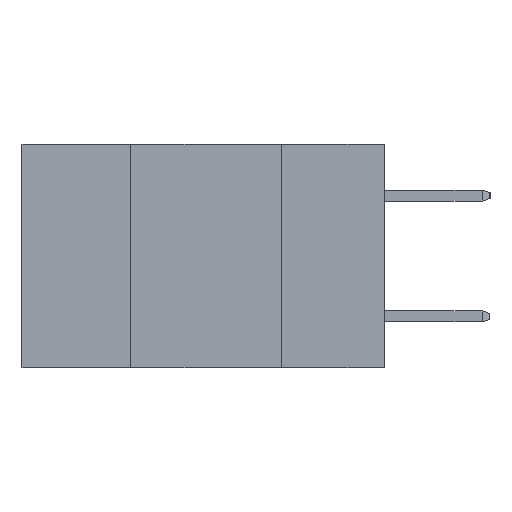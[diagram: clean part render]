
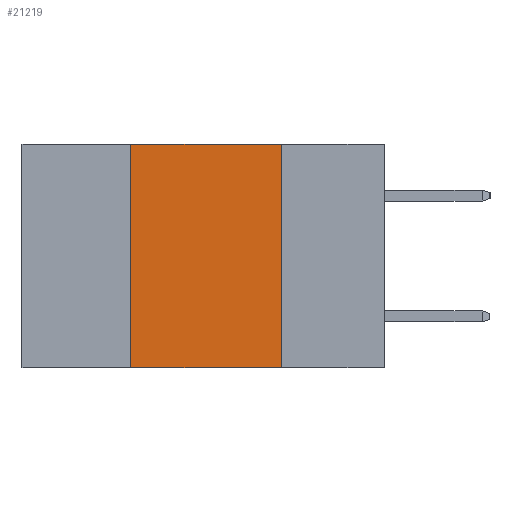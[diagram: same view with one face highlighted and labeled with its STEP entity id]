
A CAD part, left-side view. The second image highlights one B-rep face of the part: STEP entity #21219.
In plain terms, the highlighted planar face has unit normal (-1, 0, 0).
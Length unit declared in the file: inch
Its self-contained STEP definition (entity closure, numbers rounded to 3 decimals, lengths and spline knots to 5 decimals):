
#1709 = CARTESIAN_POINT ( 'NONE',  ( 0., 0.42, -0.37 ) ) ;
#1717 = VECTOR ( 'NONE', #9389, 39.37008 ) ;
#1955 = LINE ( 'NONE', #6246, #3697 ) ;
#2546 = CARTESIAN_POINT ( 'NONE',  ( 0., 0.42, -0.37 ) ) ;
#2912 = EDGE_CURVE ( 'NONE', #18429, #22947, #5205, .T. ) ;
#3544 = ORIENTED_EDGE ( 'NONE', *, *, #7092, .F. ) ;
#3697 = VECTOR ( 'NONE', #4230, 39.37008 ) ;
#3703 = CARTESIAN_POINT ( 'NONE',  ( 0., 0.17, -0.37 ) ) ;
#4230 = DIRECTION ( 'NONE',  ( 0., -1., 0. ) ) ;
#5205 = LINE ( 'NONE', #1709, #26503 ) ;
#5547 = AXIS2_PLACEMENT_3D ( 'NONE', #24723, #12268, #7936 ) ;
#6246 = CARTESIAN_POINT ( 'NONE',  ( 0., 0.6, -0.37 ) ) ;
#6876 = VERTEX_POINT ( 'NONE', #11028 ) ;
#7092 = EDGE_CURVE ( 'NONE', #6876, #13801, #21969, .T. ) ;
#7185 = EDGE_LOOP ( 'NONE', ( #3544, #21070, #16574, #25430 ) ) ;
#7936 = DIRECTION ( 'NONE',  ( 0., 0., -1. ) ) ;
#9389 = DIRECTION ( 'NONE',  ( 0., 0., -1. ) ) ;
#9823 = EDGE_CURVE ( 'NONE', #18429, #13801, #1955, .T. ) ;
#10939 = CARTESIAN_POINT ( 'NONE',  ( 0., 0.17, -0.37 ) ) ;
#11028 = CARTESIAN_POINT ( 'NONE',  ( 0., 0.17, 0. ) ) ;
#12135 = PLANE ( 'NONE',  #5547 ) ;
#12268 = DIRECTION ( 'NONE',  ( 1., 0., 0. ) ) ;
#13801 = VERTEX_POINT ( 'NONE', #10939 ) ;
#13871 = DIRECTION ( 'NONE',  ( 0., 0., 1. ) ) ;
#15457 = DIRECTION ( 'NONE',  ( 0., -1., 0. ) ) ;
#16574 = ORIENTED_EDGE ( 'NONE', *, *, #2912, .F. ) ;
#17531 = CARTESIAN_POINT ( 'NONE',  ( 0., 0.42, 0. ) ) ;
#18429 = VERTEX_POINT ( 'NONE', #2546 ) ;
#18494 = FACE_OUTER_BOUND ( 'NONE', #7185, .T. ) ;
#19924 = LINE ( 'NONE', #21426, #24640 ) ;
#21070 = ORIENTED_EDGE ( 'NONE', *, *, #23326, .F. ) ;
#21219 = ADVANCED_FACE ( 'NONE', ( #18494 ), #12135, .F. ) ;
#21426 = CARTESIAN_POINT ( 'NONE',  ( 0., 0.6, 0. ) ) ;
#21969 = LINE ( 'NONE', #3703, #1717 ) ;
#22947 = VERTEX_POINT ( 'NONE', #17531 ) ;
#23326 = EDGE_CURVE ( 'NONE', #22947, #6876, #19924, .T. ) ;
#24640 = VECTOR ( 'NONE', #15457, 39.37008 ) ;
#24723 = CARTESIAN_POINT ( 'NONE',  ( 0., 0.6, 0. ) ) ;
#25430 = ORIENTED_EDGE ( 'NONE', *, *, #9823, .T. ) ;
#26503 = VECTOR ( 'NONE', #13871, 39.37008 ) ;
